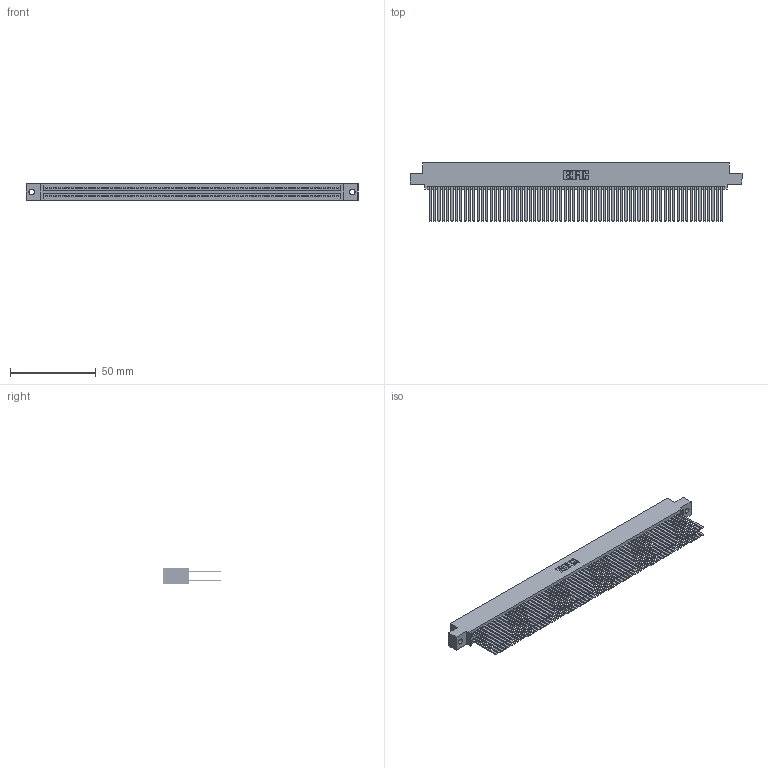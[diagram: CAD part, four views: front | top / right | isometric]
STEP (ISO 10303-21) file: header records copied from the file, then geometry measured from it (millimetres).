
FILE_DESCRIPTION (( 'STEP AP203' ), '1' );
FILE_NAME ('345-136-544-502.STEP', '2018-10-20T14:43:35', ( '' ), ( '' ), 'SwSTEP 2.0', 'SolidWorks 2016', '' );
FILE_SCHEMA (( 'CONFIG_CONTROL_DESIGN' ));
Length unit declared in the file: inch
Products named in the file (3): 345-136-544-502; 345 Part_0.110 Offset - 0.128 Dia; 345-292-001_345-293-144
Assembly tree (137 placements, depth 2):
  345-136-544-502
    345 Part_0.110 Offset - 0.128 Dia
    345-292-001_345-293-144  x136
Bounding box: 193.93 x 33.96 x 9.4 mm (x, y, z)
Volume: 20876.2 mm3; surface area: 36769.9 mm2
Topology: 137 solids, 137 shells, 6114 faces, 18169 edges, 11930 vertices
Faces by surface type: plane 4028, cylinder 2086
Entity records: 49805 total; most frequent: CARTESIAN_POINT 8324, ORIENTED_EDGE 8258, DIRECTION 7305, EDGE_CURVE 4129, VECTOR 3729, LINE 3729, VERTEX_POINT 2750, AXIS2_PLACEMENT_3D 1788
